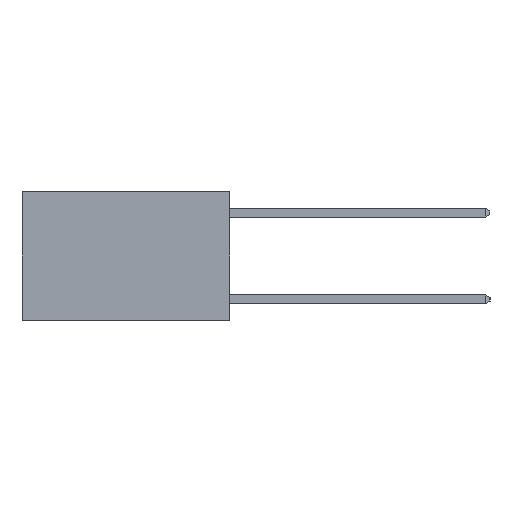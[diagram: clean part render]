
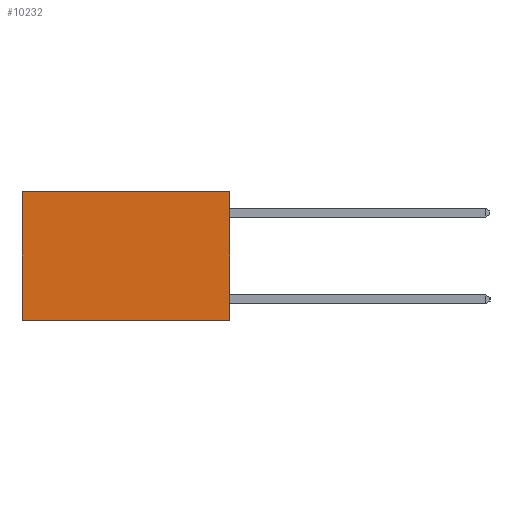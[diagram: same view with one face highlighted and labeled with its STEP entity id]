
A CAD part, left-side view. The second image highlights one B-rep face of the part: STEP entity #10232.
In plain terms, the highlighted planar face has unit normal (-1, 0, 0).
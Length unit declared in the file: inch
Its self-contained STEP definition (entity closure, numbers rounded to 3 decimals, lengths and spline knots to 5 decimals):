
#429 = CARTESIAN_POINT ( 'NONE',  ( 0.2625, 0., -0.37 ) ) ;
#485 = ORIENTED_EDGE ( 'NONE', *, *, #4641, .T. ) ;
#714 = EDGE_CURVE ( 'NONE', #6138, #3718, #1760, .T. ) ;
#952 = CARTESIAN_POINT ( 'NONE',  ( 0.2625, 0.6, 0. ) ) ;
#1017 = LINE ( 'NONE', #1517, #9261 ) ;
#1102 = CARTESIAN_POINT ( 'NONE',  ( 0.2625, 0., 0. ) ) ;
#1235 = DIRECTION ( 'NONE',  ( 0., 1., 0. ) ) ;
#1343 = VECTOR ( 'NONE', #1235, 39.37008 ) ;
#1517 = CARTESIAN_POINT ( 'NONE',  ( 0.2625, 0., 0. ) ) ;
#1760 = LINE ( 'NONE', #2136, #5724 ) ;
#1843 = EDGE_CURVE ( 'NONE', #3718, #2202, #7474, .T. ) ;
#2029 = DIRECTION ( 'NONE',  ( 0., 0., -1. ) ) ;
#2136 = CARTESIAN_POINT ( 'NONE',  ( 0.2625, 0., 0. ) ) ;
#2202 = VERTEX_POINT ( 'NONE', #2604 ) ;
#2407 = VERTEX_POINT ( 'NONE', #6858 ) ;
#2604 = CARTESIAN_POINT ( 'NONE',  ( 0.2625, 0.6, -0.37 ) ) ;
#2884 = ORIENTED_EDGE ( 'NONE', *, *, #6011, .T. ) ;
#2891 = CARTESIAN_POINT ( 'NONE',  ( 0.2625, 0., -0.37 ) ) ;
#2939 = DIRECTION ( 'NONE',  ( 0., 0., -1. ) ) ;
#3096 = VECTOR ( 'NONE', #7338, 39.37008 ) ;
#3718 = VERTEX_POINT ( 'NONE', #429 ) ;
#4641 = EDGE_CURVE ( 'NONE', #6138, #2407, #1017, .T. ) ;
#5272 = PLANE ( 'NONE',  #6495 ) ;
#5499 = EDGE_LOOP ( 'NONE', ( #2884, #6511, #5604, #485 ) ) ;
#5604 = ORIENTED_EDGE ( 'NONE', *, *, #714, .F. ) ;
#5724 = VECTOR ( 'NONE', #2029, 39.37008 ) ;
#6011 = EDGE_CURVE ( 'NONE', #2407, #2202, #7310, .T. ) ;
#6070 = CARTESIAN_POINT ( 'NONE',  ( 0.2625, 0., 0. ) ) ;
#6138 = VERTEX_POINT ( 'NONE', #1102 ) ;
#6495 = AXIS2_PLACEMENT_3D ( 'NONE', #6070, #7687, #2939 ) ;
#6511 = ORIENTED_EDGE ( 'NONE', *, *, #1843, .F. ) ;
#6858 = CARTESIAN_POINT ( 'NONE',  ( 0.2625, 0.6, 0. ) ) ;
#7310 = LINE ( 'NONE', #952, #3096 ) ;
#7338 = DIRECTION ( 'NONE',  ( 0., 0., -1. ) ) ;
#7474 = LINE ( 'NONE', #2891, #1343 ) ;
#7687 = DIRECTION ( 'NONE',  ( 1., 0., 0. ) ) ;
#8831 = FACE_OUTER_BOUND ( 'NONE', #5499, .T. ) ;
#9261 = VECTOR ( 'NONE', #9456, 39.37008 ) ;
#9456 = DIRECTION ( 'NONE',  ( 0., 1., 0. ) ) ;
#10232 = ADVANCED_FACE ( 'NONE', ( #8831 ), #5272, .F. ) ;
